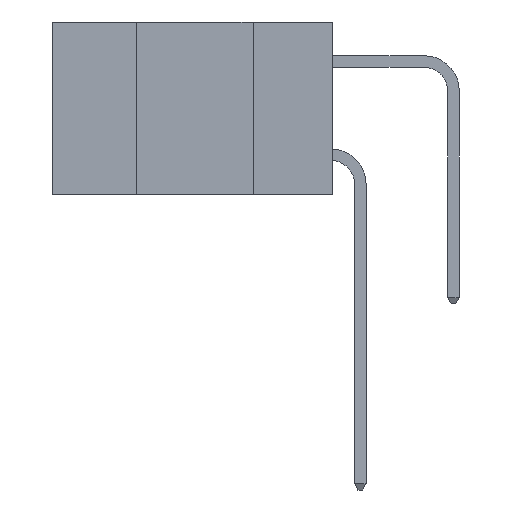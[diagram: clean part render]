
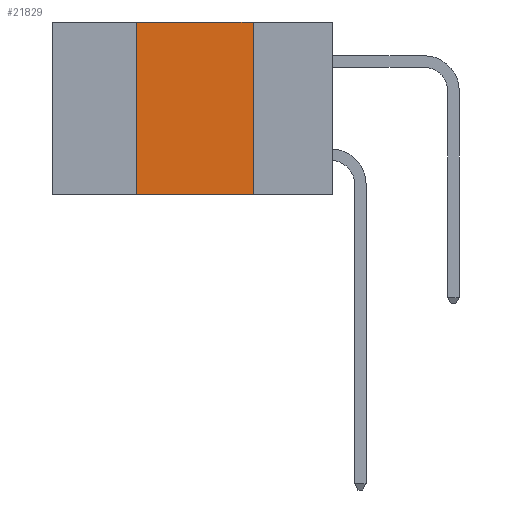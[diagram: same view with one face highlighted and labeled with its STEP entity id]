
A CAD part, left-side view. The second image highlights one B-rep face of the part: STEP entity #21829.
In plain terms, the highlighted planar face has unit normal (-1, 0, 0).
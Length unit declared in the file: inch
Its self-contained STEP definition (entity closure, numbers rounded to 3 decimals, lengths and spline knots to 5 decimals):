
#192 = EDGE_LOOP ( 'NONE', ( #21495, #2319, #8601, #13551 ) ) ;
#1055 = LINE ( 'NONE', #19632, #20290 ) ;
#1344 = VERTEX_POINT ( 'NONE', #4850 ) ;
#1805 = VECTOR ( 'NONE', #16716, 39.37008 ) ;
#2319 = ORIENTED_EDGE ( 'NONE', *, *, #12196, .F. ) ;
#2577 = LINE ( 'NONE', #13827, #12894 ) ;
#2718 = AXIS2_PLACEMENT_3D ( 'NONE', #18234, #14616, #3344 ) ;
#2926 = DIRECTION ( 'NONE',  ( 0., -1., 0. ) ) ;
#3344 = DIRECTION ( 'NONE',  ( 0., 0., -1. ) ) ;
#3575 = CARTESIAN_POINT ( 'NONE',  ( 0., 0.42, 0. ) ) ;
#4538 = LINE ( 'NONE', #22362, #23602 ) ;
#4571 = CARTESIAN_POINT ( 'NONE',  ( 0., 0.17, -0.37 ) ) ;
#4850 = CARTESIAN_POINT ( 'NONE',  ( 0., 0.42, -0.37 ) ) ;
#4881 = VERTEX_POINT ( 'NONE', #3575 ) ;
#6303 = VERTEX_POINT ( 'NONE', #15098 ) ;
#8601 = ORIENTED_EDGE ( 'NONE', *, *, #17126, .F. ) ;
#9276 = CARTESIAN_POINT ( 'NONE',  ( 0., 0.6, -0.37 ) ) ;
#12196 = EDGE_CURVE ( 'NONE', #4881, #6303, #1055, .T. ) ;
#12761 = PLANE ( 'NONE',  #2718 ) ;
#12894 = VECTOR ( 'NONE', #19342, 39.37008 ) ;
#13431 = EDGE_CURVE ( 'NONE', #6303, #15903, #4538, .T. ) ;
#13551 = ORIENTED_EDGE ( 'NONE', *, *, #14666, .T. ) ;
#13827 = CARTESIAN_POINT ( 'NONE',  ( 0., 0.42, -0.37 ) ) ;
#14616 = DIRECTION ( 'NONE',  ( 1., 0., 0. ) ) ;
#14666 = EDGE_CURVE ( 'NONE', #1344, #15903, #22117, .T. ) ;
#15098 = CARTESIAN_POINT ( 'NONE',  ( 0., 0.17, 0. ) ) ;
#15903 = VERTEX_POINT ( 'NONE', #4571 ) ;
#16716 = DIRECTION ( 'NONE',  ( 0., -1., 0. ) ) ;
#17126 = EDGE_CURVE ( 'NONE', #1344, #4881, #2577, .T. ) ;
#18234 = CARTESIAN_POINT ( 'NONE',  ( 0., 0.6, 0. ) ) ;
#18866 = DIRECTION ( 'NONE',  ( 0., 0., -1. ) ) ;
#19342 = DIRECTION ( 'NONE',  ( 0., 0., 1. ) ) ;
#19632 = CARTESIAN_POINT ( 'NONE',  ( 0., 0.6, 0. ) ) ;
#20290 = VECTOR ( 'NONE', #2926, 39.37008 ) ;
#21495 = ORIENTED_EDGE ( 'NONE', *, *, #13431, .F. ) ;
#21829 = ADVANCED_FACE ( 'NONE', ( #22605 ), #12761, .F. ) ;
#22117 = LINE ( 'NONE', #9276, #1805 ) ;
#22362 = CARTESIAN_POINT ( 'NONE',  ( 0., 0.17, -0.37 ) ) ;
#22605 = FACE_OUTER_BOUND ( 'NONE', #192, .T. ) ;
#23602 = VECTOR ( 'NONE', #18866, 39.37008 ) ;
